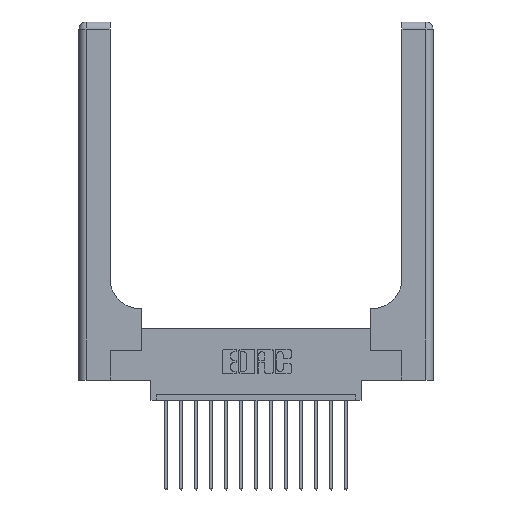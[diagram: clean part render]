
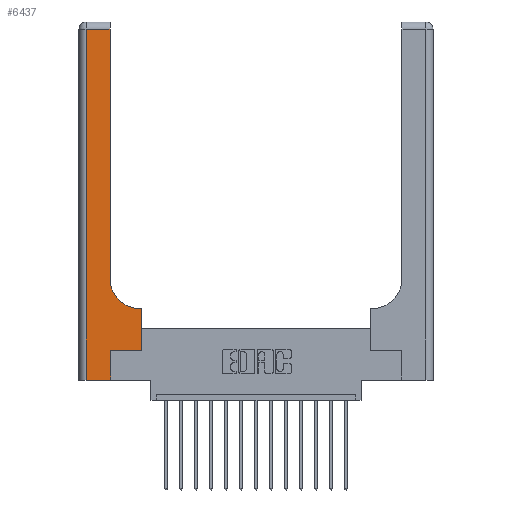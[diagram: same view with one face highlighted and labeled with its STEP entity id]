
A CAD part, top view. The second image highlights one B-rep face of the part: STEP entity #6437.
In plain terms, the highlighted planar face has unit normal (0, 0, 1).
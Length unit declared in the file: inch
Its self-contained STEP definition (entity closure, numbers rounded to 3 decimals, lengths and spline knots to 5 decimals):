
#60 = DIRECTION ( 'NONE',  ( 0., 1., 0. ) ) ;
#208 = ORIENTED_EDGE ( 'NONE', *, *, #10426, .T. ) ;
#246 = VECTOR ( 'NONE', #13773, 39.37008 ) ;
#367 = CARTESIAN_POINT ( 'NONE',  ( 0.26, 2.94, 0.37 ) ) ;
#373 = VERTEX_POINT ( 'NONE', #15899 ) ;
#456 = CARTESIAN_POINT ( 'NONE',  ( 0.26, 3., 0.37 ) ) ;
#607 = CARTESIAN_POINT ( 'NONE',  ( 0., 0., 0.37 ) ) ;
#636 = VECTOR ( 'NONE', #4089, 39.37008 ) ;
#954 = ORIENTED_EDGE ( 'NONE', *, *, #11756, .T. ) ;
#1053 = EDGE_CURVE ( 'NONE', #12514, #4239, #1701, .T. ) ;
#1120 = CARTESIAN_POINT ( 'NONE',  ( 0.51, 0.6, 0.37 ) ) ;
#1216 = DIRECTION ( 'NONE',  ( 0., 0., -1. ) ) ;
#1376 = EDGE_CURVE ( 'NONE', #4239, #7783, #5024, .T. ) ;
#1405 = DIRECTION ( 'NONE',  ( 0., -1., 0. ) ) ;
#1413 = VERTEX_POINT ( 'NONE', #9891 ) ;
#1701 = LINE ( 'NONE', #456, #15676 ) ;
#1781 = VECTOR ( 'NONE', #1405, 39.37008 ) ;
#2222 = CIRCLE ( 'NONE', #11032, 0.25 ) ;
#2317 = CARTESIAN_POINT ( 'NONE',  ( 0.528, 0.6, 0.37 ) ) ;
#2394 = CARTESIAN_POINT ( 'NONE',  ( 0.51, 0.85, 0.37 ) ) ;
#2479 = CARTESIAN_POINT ( 'NONE',  ( 0.528, 0.25, 0.37 ) ) ;
#2709 = CARTESIAN_POINT ( 'NONE',  ( 0.06, 2.94, 0.37 ) ) ;
#3010 = VERTEX_POINT ( 'NONE', #6776 ) ;
#3022 = EDGE_LOOP ( 'NONE', ( #17129, #12760, #13654, #208, #7252, #4775, #954, #12855, #8976 ) ) ;
#3221 = DIRECTION ( 'NONE',  ( 0., 1., 0. ) ) ;
#3293 = LINE ( 'NONE', #607, #4931 ) ;
#3824 = DIRECTION ( 'NONE',  ( 1., 0., 0. ) ) ;
#3851 = LINE ( 'NONE', #9241, #5108 ) ;
#4089 = DIRECTION ( 'NONE',  ( 0., 1., 0. ) ) ;
#4239 = VERTEX_POINT ( 'NONE', #367 ) ;
#4543 = DIRECTION ( 'NONE',  ( 1., 0., 0. ) ) ;
#4775 = ORIENTED_EDGE ( 'NONE', *, *, #10319, .T. ) ;
#4931 = VECTOR ( 'NONE', #11466, 39.37008 ) ;
#5024 = LINE ( 'NONE', #10422, #246 ) ;
#5108 = VECTOR ( 'NONE', #14725, 39.37008 ) ;
#5142 = PLANE ( 'NONE',  #7649 ) ;
#5535 = LINE ( 'NONE', #9418, #1781 ) ;
#5700 = LINE ( 'NONE', #8236, #8307 ) ;
#6417 = VERTEX_POINT ( 'NONE', #14632 ) ;
#6437 = ADVANCED_FACE ( 'NONE', ( #8148 ), #5142, .F. ) ;
#6776 = CARTESIAN_POINT ( 'NONE',  ( 0.265, 0., 0.37 ) ) ;
#6865 = DIRECTION ( 'NONE',  ( 0., 0., -1. ) ) ;
#7062 = EDGE_CURVE ( 'NONE', #9295, #12984, #3851, .T. ) ;
#7252 = ORIENTED_EDGE ( 'NONE', *, *, #11877, .T. ) ;
#7649 = AXIS2_PLACEMENT_3D ( 'NONE', #12001, #1216, #16015 ) ;
#7746 = VECTOR ( 'NONE', #4543, 39.37008 ) ;
#7783 = VERTEX_POINT ( 'NONE', #2709 ) ;
#8148 = FACE_OUTER_BOUND ( 'NONE', #3022, .T. ) ;
#8236 = CARTESIAN_POINT ( 'NONE',  ( 0.265, 0., 0.37 ) ) ;
#8255 = CARTESIAN_POINT ( 'NONE',  ( 0.265, 0.25, 0.37 ) ) ;
#8307 = VECTOR ( 'NONE', #60, 39.37008 ) ;
#8976 = ORIENTED_EDGE ( 'NONE', *, *, #12932, .T. ) ;
#9128 = LINE ( 'NONE', #2479, #636 ) ;
#9241 = CARTESIAN_POINT ( 'NONE',  ( 0.26, 0.6, 0.37 ) ) ;
#9295 = VERTEX_POINT ( 'NONE', #2317 ) ;
#9418 = CARTESIAN_POINT ( 'NONE',  ( 0.06, 3., 0.37 ) ) ;
#9862 = LINE ( 'NONE', #8255, #7746 ) ;
#9891 = CARTESIAN_POINT ( 'NONE',  ( 0.06, 0., 0.37 ) ) ;
#10319 = EDGE_CURVE ( 'NONE', #373, #6417, #9862, .T. ) ;
#10422 = CARTESIAN_POINT ( 'NONE',  ( 0., 2.94, 0.37 ) ) ;
#10426 = EDGE_CURVE ( 'NONE', #1413, #3010, #3293, .T. ) ;
#10952 = CARTESIAN_POINT ( 'NONE',  ( 0.26, 0.85, 0.37 ) ) ;
#11032 = AXIS2_PLACEMENT_3D ( 'NONE', #2394, #6865, #3824 ) ;
#11466 = DIRECTION ( 'NONE',  ( 1., 0., 0. ) ) ;
#11756 = EDGE_CURVE ( 'NONE', #6417, #9295, #9128, .T. ) ;
#11877 = EDGE_CURVE ( 'NONE', #3010, #373, #5700, .T. ) ;
#12001 = CARTESIAN_POINT ( 'NONE',  ( 0., 3., 0.37 ) ) ;
#12514 = VERTEX_POINT ( 'NONE', #10952 ) ;
#12760 = ORIENTED_EDGE ( 'NONE', *, *, #1376, .T. ) ;
#12855 = ORIENTED_EDGE ( 'NONE', *, *, #7062, .T. ) ;
#12932 = EDGE_CURVE ( 'NONE', #12984, #12514, #2222, .T. ) ;
#12984 = VERTEX_POINT ( 'NONE', #1120 ) ;
#13654 = ORIENTED_EDGE ( 'NONE', *, *, #15120, .T. ) ;
#13773 = DIRECTION ( 'NONE',  ( -1., 0., 0. ) ) ;
#14632 = CARTESIAN_POINT ( 'NONE',  ( 0.528, 0.25, 0.37 ) ) ;
#14725 = DIRECTION ( 'NONE',  ( -1., 0., 0. ) ) ;
#15120 = EDGE_CURVE ( 'NONE', #7783, #1413, #5535, .T. ) ;
#15676 = VECTOR ( 'NONE', #3221, 39.37008 ) ;
#15899 = CARTESIAN_POINT ( 'NONE',  ( 0.265, 0.25, 0.37 ) ) ;
#16015 = DIRECTION ( 'NONE',  ( -1., 0., 0. ) ) ;
#17129 = ORIENTED_EDGE ( 'NONE', *, *, #1053, .T. ) ;
